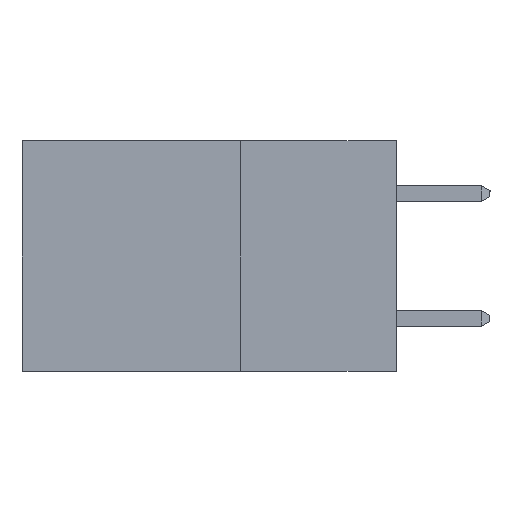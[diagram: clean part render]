
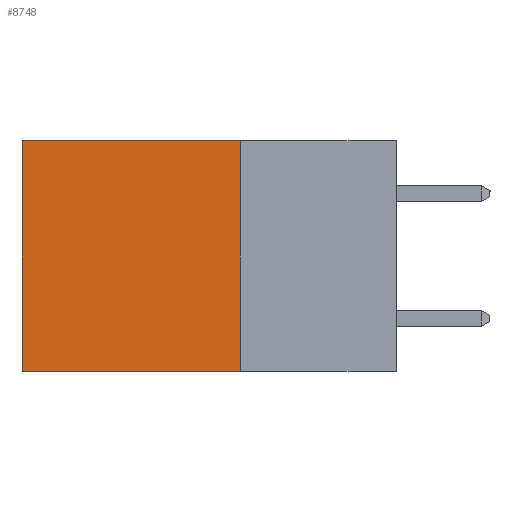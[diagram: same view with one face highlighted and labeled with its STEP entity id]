
A CAD part, left-side view. The second image highlights one B-rep face of the part: STEP entity #8748.
In plain terms, the highlighted planar face has unit normal (-1, 0, 0).
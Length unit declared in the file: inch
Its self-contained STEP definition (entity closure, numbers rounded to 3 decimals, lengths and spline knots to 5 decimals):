
#462 = CARTESIAN_POINT ( 'NONE',  ( 0.2615, 0.25, -0.37 ) ) ;
#767 = ORIENTED_EDGE ( 'NONE', *, *, #5832, .T. ) ;
#994 = DIRECTION ( 'NONE',  ( 0., 0., -1. ) ) ;
#1181 = VECTOR ( 'NONE', #8417, 39.37008 ) ;
#2214 = CARTESIAN_POINT ( 'NONE',  ( 0.2615, 0.25, 0. ) ) ;
#2550 = VERTEX_POINT ( 'NONE', #7248 ) ;
#2759 = VECTOR ( 'NONE', #3514, 39.37008 ) ;
#3514 = DIRECTION ( 'NONE',  ( 0., 1., 0. ) ) ;
#4397 = CARTESIAN_POINT ( 'NONE',  ( 0.2615, 0.25, -0.37 ) ) ;
#4682 = ORIENTED_EDGE ( 'NONE', *, *, #12148, .F. ) ;
#5101 = CARTESIAN_POINT ( 'NONE',  ( 0.2615, 0.6, -0.37 ) ) ;
#5284 = CARTESIAN_POINT ( 'NONE',  ( 0.2615, 0.6, 0. ) ) ;
#5320 = VERTEX_POINT ( 'NONE', #7028 ) ;
#5832 = EDGE_CURVE ( 'NONE', #13098, #2550, #18904, .T. ) ;
#6239 = EDGE_LOOP ( 'NONE', ( #767, #4682, #13193, #7481 ) ) ;
#6728 = VERTEX_POINT ( 'NONE', #19029 ) ;
#7028 = CARTESIAN_POINT ( 'NONE',  ( 0.2615, 0.25, 0. ) ) ;
#7248 = CARTESIAN_POINT ( 'NONE',  ( 0.2615, 0.6, -0.37 ) ) ;
#7414 = LINE ( 'NONE', #4397, #18315 ) ;
#7481 = ORIENTED_EDGE ( 'NONE', *, *, #17467, .T. ) ;
#8417 = DIRECTION ( 'NONE',  ( 0., 0., -1. ) ) ;
#8748 = ADVANCED_FACE ( 'NONE', ( #15358 ), #17176, .F. ) ;
#9849 = LINE ( 'NONE', #2214, #2759 ) ;
#10117 = DIRECTION ( 'NONE',  ( 0., 1., 0. ) ) ;
#11527 = LINE ( 'NONE', #14849, #15122 ) ;
#11587 = EDGE_CURVE ( 'NONE', #5320, #6728, #7414, .T. ) ;
#12148 = EDGE_CURVE ( 'NONE', #6728, #2550, #11527, .T. ) ;
#13098 = VERTEX_POINT ( 'NONE', #5284 ) ;
#13193 = ORIENTED_EDGE ( 'NONE', *, *, #11587, .F. ) ;
#13930 = DIRECTION ( 'NONE',  ( 0., 0., -1. ) ) ;
#14849 = CARTESIAN_POINT ( 'NONE',  ( 0.2615, 0.25, -0.37 ) ) ;
#15122 = VECTOR ( 'NONE', #10117, 39.37008 ) ;
#15358 = FACE_OUTER_BOUND ( 'NONE', #6239, .T. ) ;
#15798 = AXIS2_PLACEMENT_3D ( 'NONE', #462, #17075, #13930 ) ;
#17075 = DIRECTION ( 'NONE',  ( 1., 0., 0. ) ) ;
#17176 = PLANE ( 'NONE',  #15798 ) ;
#17467 = EDGE_CURVE ( 'NONE', #5320, #13098, #9849, .T. ) ;
#18315 = VECTOR ( 'NONE', #994, 39.37008 ) ;
#18904 = LINE ( 'NONE', #5101, #1181 ) ;
#19029 = CARTESIAN_POINT ( 'NONE',  ( 0.2615, 0.25, -0.37 ) ) ;
